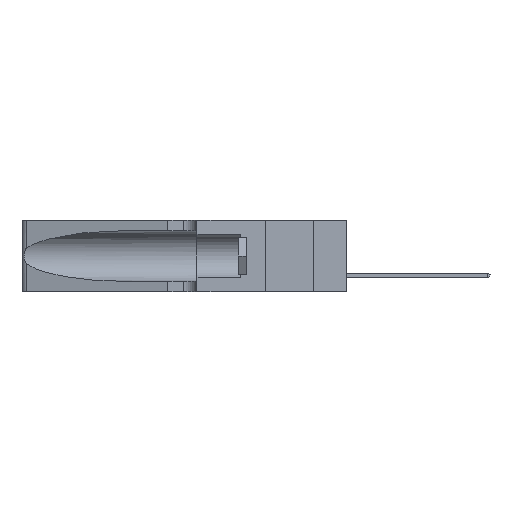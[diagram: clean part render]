
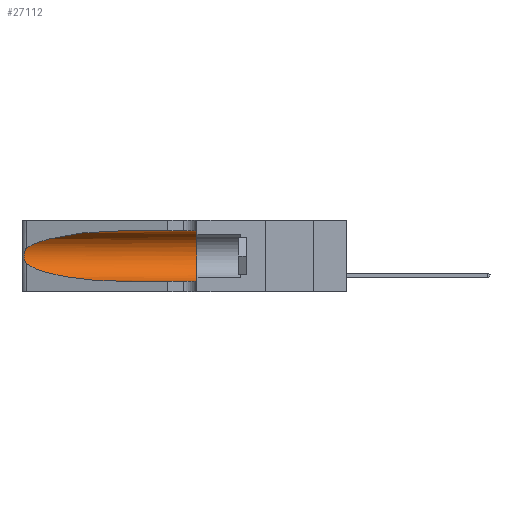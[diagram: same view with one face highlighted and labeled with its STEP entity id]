
A CAD part, left-side view. The second image highlights one B-rep face of the part: STEP entity #27112.
In plain terms, the highlighted cylindrical face has radius 3.308 mm (diameter 6.617 mm), a partial arc.
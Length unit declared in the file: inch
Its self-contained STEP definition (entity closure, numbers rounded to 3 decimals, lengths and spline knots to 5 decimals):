
#8 = DIRECTION ( 'NONE',  ( 0., -1., 0. ) ) ;
#306 = CARTESIAN_POINT ( 'NONE',  ( 0.25555, 1.22993, 0.14849 ) ) ;
#2131 = CARTESIAN_POINT ( 'NONE',  ( 0.1305, 0.72297, 0.05475 ) ) ;
#2593 = ORIENTED_EDGE ( 'NONE', *, *, #25062, .T. ) ;
#2596 = CARTESIAN_POINT ( 'NONE',  ( 0.25487, 1.22718, 0.14631 ) ) ;
#2678 = VERTEX_POINT ( 'NONE', #27285 ) ;
#3210 = EDGE_CURVE ( 'NONE', #15588, #10808, #6942, .T. ) ;
#3225 = FACE_OUTER_BOUND ( 'NONE', #8456, .T. ) ;
#3362 = CARTESIAN_POINT ( 'NONE',  ( 0.25487, 1.22718, 0.22369 ) ) ;
#4748 = CARTESIAN_POINT ( 'NONE',  ( 0.1305, 0.72297, 0.31525 ) ) ;
#4828 = CARTESIAN_POINT ( 'NONE',  ( 0.1305, 0.72297, 0.05475 ) ) ;
#4941 = DIRECTION ( 'NONE',  ( 0., 0., -1. ) ) ;
#5016 = CARTESIAN_POINT ( 'NONE',  ( 0.2373, 1.15595, 0.08982 ) ) ;
#5339 = CARTESIAN_POINT ( 'NONE',  ( 0.18966, 0.96281, 0.31525 ) ) ;
#6686 = CARTESIAN_POINT ( 'NONE',  ( 0.1305, 1.61858, 0.05475 ) ) ;
#6942 = LINE ( 'NONE', #26770, #13414 ) ;
#7103 = CARTESIAN_POINT ( 'NONE',  ( 0.25639, 1.23184, 0.21858 ) ) ;
#8273 = VECTOR ( 'NONE', #8, 39.37008 ) ;
#8456 = EDGE_LOOP ( 'NONE', ( #15930, #21553, #18475, #2593, #24596, #25478 ) ) ;
#8612 = LINE ( 'NONE', #6686, #8273 ) ;
#9013 = CARTESIAN_POINT ( 'NONE',  ( 0.25555, 1.22994, 0.2215 ) ) ;
#9029 = AXIS2_PLACEMENT_3D ( 'NONE', #9797, #19718, #10601 ) ;
#9387 = CARTESIAN_POINT ( 'NONE',  ( 0.25854, 1.2359, 0.20912 ) ) ;
#9797 = CARTESIAN_POINT ( 'NONE',  ( 0.1305, 0.35, 0.185 ) ) ;
#10201 = CIRCLE ( 'NONE', #9029, 0.13025 ) ;
#10601 = DIRECTION ( 'NONE',  ( 0., 0., 1. ) ) ;
#10735 = CYLINDRICAL_SURFACE ( 'NONE', #15342, 0.13025 ) ;
#10808 = VERTEX_POINT ( 'NONE', #18875 ) ;
#11015 = VERTEX_POINT ( 'NONE', #16645 ) ;
#11299 = CARTESIAN_POINT ( 'NONE',  ( 0.25856, 1.23593, 0.16098 ) ) ;
#11607 = EDGE_CURVE ( 'NONE', #15588, #11015, #16444, .T. ) ;
#11672 = CARTESIAN_POINT ( 'NONE',  ( 0.25789, 1.23486, 0.15765 ) ) ;
#12432 = B_SPLINE_CURVE_WITH_KNOTS ( 'NONE', 3,
 ( #27572, #9013, #7103, #18495, #9387, #16289, #18216, #16006, #25370, #11299, #11672, #13995, #306, #2596 ),
 .UNSPECIFIED., .F., .F.,
 ( 4, 2, 2, 2, 2, 2, 4 ),
 ( 0., 0.00027, 0.00053, 0.00107, 0.0016, 0.00187, 0.00214 ),
 .UNSPECIFIED. ) ;
#13043 = VERTEX_POINT ( 'NONE', #2131 ) ;
#13414 = VECTOR ( 'NONE', #29089, 39.37008 ) ;
#13995 = CARTESIAN_POINT ( 'NONE',  ( 0.25639, 1.23186, 0.15144 ) ) ;
#15073 = VERTEX_POINT ( 'NONE', #29558 ) ;
#15342 = AXIS2_PLACEMENT_3D ( 'NONE', #19070, #25824, #4941 ) ;
#15437 = EDGE_CURVE ( 'NONE', #15073, #13043, #22167, .T. ) ;
#15588 = VERTEX_POINT ( 'NONE', #28173 ) ;
#15930 = ORIENTED_EDGE ( 'NONE', *, *, #11607, .T. ) ;
#16006 = CARTESIAN_POINT ( 'NONE',  ( 0.26075, 1.23896, 0.178 ) ) ;
#16289 = CARTESIAN_POINT ( 'NONE',  ( 0.26018, 1.23835, 0.19895 ) ) ;
#16444 =( BOUNDED_CURVE ( )  B_SPLINE_CURVE ( 3, ( #4748, #5339, #21305, #3362 ),
 .UNSPECIFIED., .F., .F. ) 
 B_SPLINE_CURVE_WITH_KNOTS ( ( 4, 4 ),
 ( 1.5708, 2.84003 ),
 .UNSPECIFIED. ) 
 CURVE ( )  GEOMETRIC_REPRESENTATION_ITEM ( )  RATIONAL_B_SPLINE_CURVE ( ( 1., 0.87, 0.87, 1. ) ) 
 REPRESENTATION_ITEM ( '' )  );
#16645 = CARTESIAN_POINT ( 'NONE',  ( 0.25487, 1.22718, 0.22369 ) ) ;
#18167 = EDGE_CURVE ( 'NONE', #10808, #2678, #10201, .T. ) ;
#18216 = CARTESIAN_POINT ( 'NONE',  ( 0.26075, 1.23896, 0.19203 ) ) ;
#18475 = ORIENTED_EDGE ( 'NONE', *, *, #15437, .T. ) ;
#18495 = CARTESIAN_POINT ( 'NONE',  ( 0.25787, 1.23484, 0.2124 ) ) ;
#18730 = CARTESIAN_POINT ( 'NONE',  ( 0.25487, 1.22718, 0.14631 ) ) ;
#18875 = CARTESIAN_POINT ( 'NONE',  ( 0.1305, 0.35, 0.31525 ) ) ;
#19070 = CARTESIAN_POINT ( 'NONE',  ( 0.1305, 1.61858, 0.185 ) ) ;
#19718 = DIRECTION ( 'NONE',  ( 0., 1., 0. ) ) ;
#21305 = CARTESIAN_POINT ( 'NONE',  ( 0.2373, 1.15595, 0.28018 ) ) ;
#21553 = ORIENTED_EDGE ( 'NONE', *, *, #22060, .T. ) ;
#22060 = EDGE_CURVE ( 'NONE', #11015, #15073, #12432, .T. ) ;
#22167 =( BOUNDED_CURVE ( )  B_SPLINE_CURVE ( 3, ( #18730, #5016, #25799, #4828 ),
 .UNSPECIFIED., .F., .T. ) 
 B_SPLINE_CURVE_WITH_KNOTS ( ( 4, 4 ),
 ( 3.44316, 4.71239 ),
 .UNSPECIFIED. ) 
 CURVE ( )  GEOMETRIC_REPRESENTATION_ITEM ( )  RATIONAL_B_SPLINE_CURVE ( ( 1., 0.87, 0.87, 1. ) ) 
 REPRESENTATION_ITEM ( '' )  );
#24596 = ORIENTED_EDGE ( 'NONE', *, *, #18167, .F. ) ;
#25062 = EDGE_CURVE ( 'NONE', #13043, #2678, #8612, .T. ) ;
#25370 = CARTESIAN_POINT ( 'NONE',  ( 0.26017, 1.23833, 0.17102 ) ) ;
#25478 = ORIENTED_EDGE ( 'NONE', *, *, #3210, .F. ) ;
#25799 = CARTESIAN_POINT ( 'NONE',  ( 0.18966, 0.96281, 0.05475 ) ) ;
#25824 = DIRECTION ( 'NONE',  ( 0., -1., 0. ) ) ;
#26770 = CARTESIAN_POINT ( 'NONE',  ( 0.1305, 1.61858, 0.31525 ) ) ;
#27112 = ADVANCED_FACE ( 'NONE', ( #3225 ), #10735, .F. ) ;
#27285 = CARTESIAN_POINT ( 'NONE',  ( 0.1305, 0.35, 0.05475 ) ) ;
#27572 = CARTESIAN_POINT ( 'NONE',  ( 0.25487, 1.22718, 0.22369 ) ) ;
#28173 = CARTESIAN_POINT ( 'NONE',  ( 0.1305, 0.72297, 0.31525 ) ) ;
#29089 = DIRECTION ( 'NONE',  ( 0., -1., 0. ) ) ;
#29558 = CARTESIAN_POINT ( 'NONE',  ( 0.25487, 1.22718, 0.14631 ) ) ;
